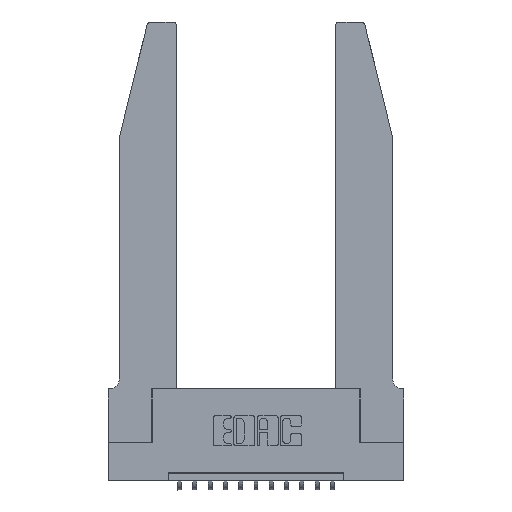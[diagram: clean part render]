
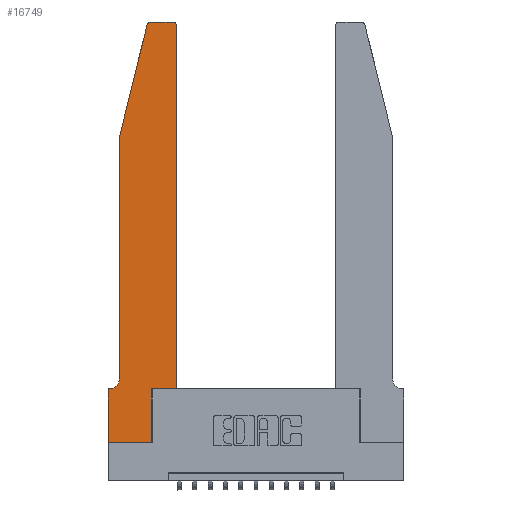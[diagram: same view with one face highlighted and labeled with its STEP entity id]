
A CAD part, top view. The second image highlights one B-rep face of the part: STEP entity #16749.
In plain terms, the highlighted planar face has unit normal (0, 0, 1).
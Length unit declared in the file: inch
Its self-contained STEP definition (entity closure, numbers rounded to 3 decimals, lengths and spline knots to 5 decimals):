
#381 = EDGE_CURVE ( 'NONE', #16378, #8747, #16802, .T. ) ;
#692 = ORIENTED_EDGE ( 'NONE', *, *, #8611, .T. ) ;
#1120 = VERTEX_POINT ( 'NONE', #6311 ) ;
#1177 = PLANE ( 'NONE',  #5084 ) ;
#1213 = EDGE_CURVE ( 'NONE', #8747, #1528, #15983, .T. ) ;
#1232 = DIRECTION ( 'NONE',  ( 0., 0., 1. ) ) ;
#1262 = CARTESIAN_POINT ( 'NONE',  ( 0., 0.35, 0.37 ) ) ;
#1337 = LINE ( 'NONE', #15144, #14874 ) ;
#1440 = EDGE_CURVE ( 'NONE', #5229, #3955, #4060, .T. ) ;
#1476 = ORIENTED_EDGE ( 'NONE', *, *, #1440, .T. ) ;
#1528 = VERTEX_POINT ( 'NONE', #2533 ) ;
#1632 = CARTESIAN_POINT ( 'NONE',  ( 0.2865, 0., 0.37 ) ) ;
#1932 = CARTESIAN_POINT ( 'NONE',  ( 0.0755, 2., 0.37 ) ) ;
#2230 = DIRECTION ( 'NONE',  ( 1., 0., 0. ) ) ;
#2247 = LINE ( 'NONE', #6155, #16029 ) ;
#2508 = DIRECTION ( 'NONE',  ( -1., 0., 0. ) ) ;
#2533 = CARTESIAN_POINT ( 'NONE',  ( 0.4505, 0.35, 0.37 ) ) ;
#2772 = DIRECTION ( 'NONE',  ( 0., 1., 0. ) ) ;
#2892 = DIRECTION ( 'NONE',  ( -1., 0., 0. ) ) ;
#3767 = DIRECTION ( 'NONE',  ( 1., 0., 0. ) ) ;
#3955 = VERTEX_POINT ( 'NONE', #1262 ) ;
#4060 = LINE ( 'NONE', #9842, #7200 ) ;
#4134 = VERTEX_POINT ( 'NONE', #17107 ) ;
#4273 = VECTOR ( 'NONE', #3767, 39.37008 ) ;
#4294 = CARTESIAN_POINT ( 'NONE',  ( 0.284, 2.72, 0.37 ) ) ;
#4541 = DIRECTION ( 'NONE',  ( 0., 0., 1. ) ) ;
#5084 = AXIS2_PLACEMENT_3D ( 'NONE', #10486, #1232, #5293 ) ;
#5104 = CIRCLE ( 'NONE', #13363, 0.03 ) ;
#5229 = VERTEX_POINT ( 'NONE', #8366 ) ;
#5293 = DIRECTION ( 'NONE',  ( 1., 0., 0. ) ) ;
#5454 = ORIENTED_EDGE ( 'NONE', *, *, #13510, .T. ) ;
#5472 = LINE ( 'NONE', #7935, #10693 ) ;
#5683 = DIRECTION ( 'NONE',  ( -1., 0., 0. ) ) ;
#5723 = DIRECTION ( 'NONE',  ( 0., -1., 0. ) ) ;
#5750 = DIRECTION ( 'NONE',  ( 1., 0., 0. ) ) ;
#5784 = ORIENTED_EDGE ( 'NONE', *, *, #10371, .T. ) ;
#5881 = CARTESIAN_POINT ( 'NONE',  ( 0., 0., 0.37 ) ) ;
#6155 = CARTESIAN_POINT ( 'NONE',  ( 0., 0., 0.37 ) ) ;
#6311 = CARTESIAN_POINT ( 'NONE',  ( 0.25487, 2.72718, 0.37 ) ) ;
#6344 = CARTESIAN_POINT ( 'NONE',  ( 0.4505, 0.35, 0.37 ) ) ;
#6400 = LINE ( 'NONE', #6344, #13494 ) ;
#6463 = ORIENTED_EDGE ( 'NONE', *, *, #1213, .T. ) ;
#6822 = CIRCLE ( 'NONE', #13102, 0.07 ) ;
#7200 = VECTOR ( 'NONE', #5683, 39.37008 ) ;
#7276 = CARTESIAN_POINT ( 'NONE',  ( 0.0755, 2., 0.37 ) ) ;
#7818 = FACE_OUTER_BOUND ( 'NONE', #13659, .T. ) ;
#7935 = CARTESIAN_POINT ( 'NONE',  ( 0.2605, 2.75, 0.37 ) ) ;
#8366 = CARTESIAN_POINT ( 'NONE',  ( 0.0055, 0.35, 0.37 ) ) ;
#8611 = EDGE_CURVE ( 'NONE', #1120, #14607, #16937, .T. ) ;
#8747 = VERTEX_POINT ( 'NONE', #14366 ) ;
#8860 = DIRECTION ( 'NONE',  ( 1., 0., 0. ) ) ;
#8916 = LINE ( 'NONE', #7276, #16224 ) ;
#8996 = CARTESIAN_POINT ( 'NONE',  ( 0.4205, 2.72, 0.37 ) ) ;
#9373 = CARTESIAN_POINT ( 'NONE',  ( 0.4205, 2.75, 0.37 ) ) ;
#9732 = ORIENTED_EDGE ( 'NONE', *, *, #11049, .T. ) ;
#9842 = CARTESIAN_POINT ( 'NONE',  ( 0.0755, 0.35, 0.37 ) ) ;
#10371 = EDGE_CURVE ( 'NONE', #3955, #12661, #2247, .T. ) ;
#10486 = CARTESIAN_POINT ( 'NONE',  ( 0., 0.35, 0.37 ) ) ;
#10593 = EDGE_CURVE ( 'NONE', #1528, #12187, #6400, .T. ) ;
#10613 = VERTEX_POINT ( 'NONE', #9373 ) ;
#10693 = VECTOR ( 'NONE', #2508, 39.37008 ) ;
#10747 = ORIENTED_EDGE ( 'NONE', *, *, #13155, .T. ) ;
#10921 = DIRECTION ( 'NONE',  ( 0., 0., -1. ) ) ;
#10980 = DIRECTION ( 'NONE',  ( 0., -1., 0. ) ) ;
#11049 = EDGE_CURVE ( 'NONE', #4134, #1120, #15621, .T. ) ;
#11498 = DIRECTION ( 'NONE',  ( 0., 0., 1. ) ) ;
#11500 = EDGE_CURVE ( 'NONE', #15489, #5229, #6822, .T. ) ;
#11710 = EDGE_CURVE ( 'NONE', #14607, #15489, #8916, .T. ) ;
#11753 = CARTESIAN_POINT ( 'NONE',  ( 0.4505, 0.35, 0.37 ) ) ;
#11769 = CARTESIAN_POINT ( 'NONE',  ( 0.4505, 2.72, 0.37 ) ) ;
#11787 = ORIENTED_EDGE ( 'NONE', *, *, #16572, .T. ) ;
#12187 = VERTEX_POINT ( 'NONE', #11769 ) ;
#12661 = VERTEX_POINT ( 'NONE', #5881 ) ;
#12823 = DIRECTION ( 'NONE',  ( -0.239, -0.971, 0. ) ) ;
#13102 = AXIS2_PLACEMENT_3D ( 'NONE', #16042, #10921, #2892 ) ;
#13155 = EDGE_CURVE ( 'NONE', #12661, #16378, #1337, .T. ) ;
#13251 = VECTOR ( 'NONE', #16106, 39.37008 ) ;
#13363 = AXIS2_PLACEMENT_3D ( 'NONE', #8996, #11498, #2230 ) ;
#13373 = ORIENTED_EDGE ( 'NONE', *, *, #11500, .T. ) ;
#13374 = VECTOR ( 'NONE', #12823, 39.37008 ) ;
#13494 = VECTOR ( 'NONE', #2772, 39.37008 ) ;
#13510 = EDGE_CURVE ( 'NONE', #10613, #4134, #5472, .T. ) ;
#13640 = ORIENTED_EDGE ( 'NONE', *, *, #10593, .T. ) ;
#13659 = EDGE_LOOP ( 'NONE', ( #5454, #9732, #692, #17156, #13373, #1476, #5784, #10747, #15357, #6463, #13640, #11787 ) ) ;
#14366 = CARTESIAN_POINT ( 'NONE',  ( 0.2865, 0.35, 0.37 ) ) ;
#14375 = CARTESIAN_POINT ( 'NONE',  ( 0.0755, 2., 0.37 ) ) ;
#14607 = VERTEX_POINT ( 'NONE', #14375 ) ;
#14874 = VECTOR ( 'NONE', #5750, 39.37008 ) ;
#15144 = CARTESIAN_POINT ( 'NONE',  ( 0., 0., 0.37 ) ) ;
#15357 = ORIENTED_EDGE ( 'NONE', *, *, #381, .T. ) ;
#15489 = VERTEX_POINT ( 'NONE', #16922 ) ;
#15621 = CIRCLE ( 'NONE', #16667, 0.03 ) ;
#15983 = LINE ( 'NONE', #11753, #4273 ) ;
#16029 = VECTOR ( 'NONE', #10980, 39.37008 ) ;
#16042 = CARTESIAN_POINT ( 'NONE',  ( 0.0055, 0.42, 0.37 ) ) ;
#16106 = DIRECTION ( 'NONE',  ( 0., 1., 0. ) ) ;
#16155 = CARTESIAN_POINT ( 'NONE',  ( 0.2865, 0.35, 0.37 ) ) ;
#16224 = VECTOR ( 'NONE', #5723, 39.37008 ) ;
#16378 = VERTEX_POINT ( 'NONE', #1632 ) ;
#16572 = EDGE_CURVE ( 'NONE', #12187, #10613, #5104, .T. ) ;
#16667 = AXIS2_PLACEMENT_3D ( 'NONE', #4294, #4541, #8860 ) ;
#16749 = ADVANCED_FACE ( 'NONE', ( #7818 ), #1177, .T. ) ;
#16802 = LINE ( 'NONE', #16155, #13251 ) ;
#16922 = CARTESIAN_POINT ( 'NONE',  ( 0.0755, 0.42, 0.37 ) ) ;
#16937 = LINE ( 'NONE', #1932, #13374 ) ;
#17107 = CARTESIAN_POINT ( 'NONE',  ( 0.284, 2.75, 0.37 ) ) ;
#17156 = ORIENTED_EDGE ( 'NONE', *, *, #11710, .T. ) ;
